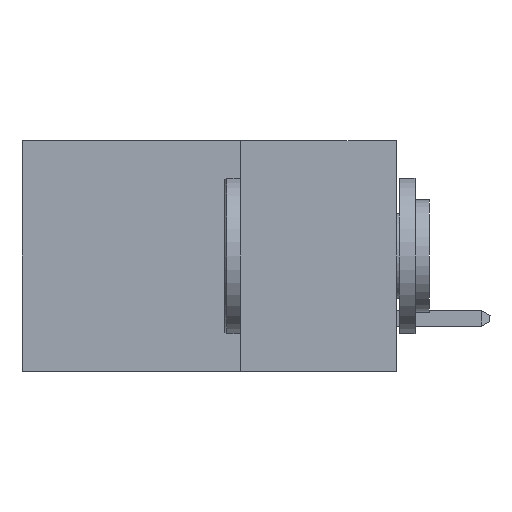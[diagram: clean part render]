
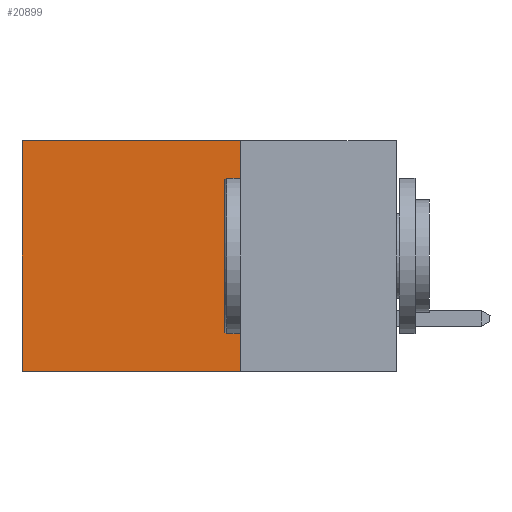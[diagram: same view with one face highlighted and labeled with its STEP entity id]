
A CAD part, left-side view. The second image highlights one B-rep face of the part: STEP entity #20899.
In plain terms, the highlighted planar face has unit normal (-1, 0, 0).
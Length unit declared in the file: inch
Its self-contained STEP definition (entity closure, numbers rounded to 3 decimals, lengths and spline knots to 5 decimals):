
#99 = VECTOR ( 'NONE', #17377, 39.37008 ) ;
#204 = PLANE ( 'NONE',  #14621 ) ;
#547 = DIRECTION ( 'NONE',  ( 1., 0., 0. ) ) ;
#795 = EDGE_CURVE ( 'NONE', #14009, #7045, #5368, .T. ) ;
#1592 = CARTESIAN_POINT ( 'NONE',  ( 0.298, 0.25, 0. ) ) ;
#2457 = DIRECTION ( 'NONE',  ( 0., 0., -1. ) ) ;
#2614 = FACE_OUTER_BOUND ( 'NONE', #4481, .T. ) ;
#2766 = CARTESIAN_POINT ( 'NONE',  ( 0.298, 0.6, 0. ) ) ;
#3118 = EDGE_CURVE ( 'NONE', #7045, #4485, #4984, .T. ) ;
#3734 = DIRECTION ( 'NONE',  ( 0., 0., -1. ) ) ;
#4481 = EDGE_LOOP ( 'NONE', ( #13229, #11903, #7721, #19541 ) ) ;
#4485 = VERTEX_POINT ( 'NONE', #8940 ) ;
#4984 = LINE ( 'NONE', #16763, #15328 ) ;
#5333 = DIRECTION ( 'NONE',  ( 0., 1., 0. ) ) ;
#5368 = LINE ( 'NONE', #1592, #8615 ) ;
#5375 = VECTOR ( 'NONE', #3734, 39.37008 ) ;
#7045 = VERTEX_POINT ( 'NONE', #23312 ) ;
#7186 = VERTEX_POINT ( 'NONE', #2766 ) ;
#7381 = EDGE_CURVE ( 'NONE', #7186, #4485, #20484, .T. ) ;
#7721 = ORIENTED_EDGE ( 'NONE', *, *, #795, .F. ) ;
#8615 = VECTOR ( 'NONE', #18769, 39.37008 ) ;
#8940 = CARTESIAN_POINT ( 'NONE',  ( 0.298, 0.6, -0.37 ) ) ;
#11276 = CARTESIAN_POINT ( 'NONE',  ( 0.298, 0.25, 0. ) ) ;
#11903 = ORIENTED_EDGE ( 'NONE', *, *, #3118, .F. ) ;
#13229 = ORIENTED_EDGE ( 'NONE', *, *, #7381, .T. ) ;
#14009 = VERTEX_POINT ( 'NONE', #11276 ) ;
#14548 = EDGE_CURVE ( 'NONE', #14009, #7186, #24101, .T. ) ;
#14621 = AXIS2_PLACEMENT_3D ( 'NONE', #17637, #547, #2457 ) ;
#14979 = CARTESIAN_POINT ( 'NONE',  ( 0.298, 0.25, 0. ) ) ;
#15088 = CARTESIAN_POINT ( 'NONE',  ( 0.298, 0.6, 0. ) ) ;
#15328 = VECTOR ( 'NONE', #5333, 39.37008 ) ;
#16763 = CARTESIAN_POINT ( 'NONE',  ( 0.298, 0.25, -0.37 ) ) ;
#17377 = DIRECTION ( 'NONE',  ( 0., 1., 0. ) ) ;
#17637 = CARTESIAN_POINT ( 'NONE',  ( 0.298, 0.25, 0. ) ) ;
#18769 = DIRECTION ( 'NONE',  ( 0., 0., -1. ) ) ;
#19541 = ORIENTED_EDGE ( 'NONE', *, *, #14548, .T. ) ;
#20484 = LINE ( 'NONE', #15088, #5375 ) ;
#20899 = ADVANCED_FACE ( 'NONE', ( #2614 ), #204, .F. ) ;
#23312 = CARTESIAN_POINT ( 'NONE',  ( 0.298, 0.25, -0.37 ) ) ;
#24101 = LINE ( 'NONE', #14979, #99 ) ;
